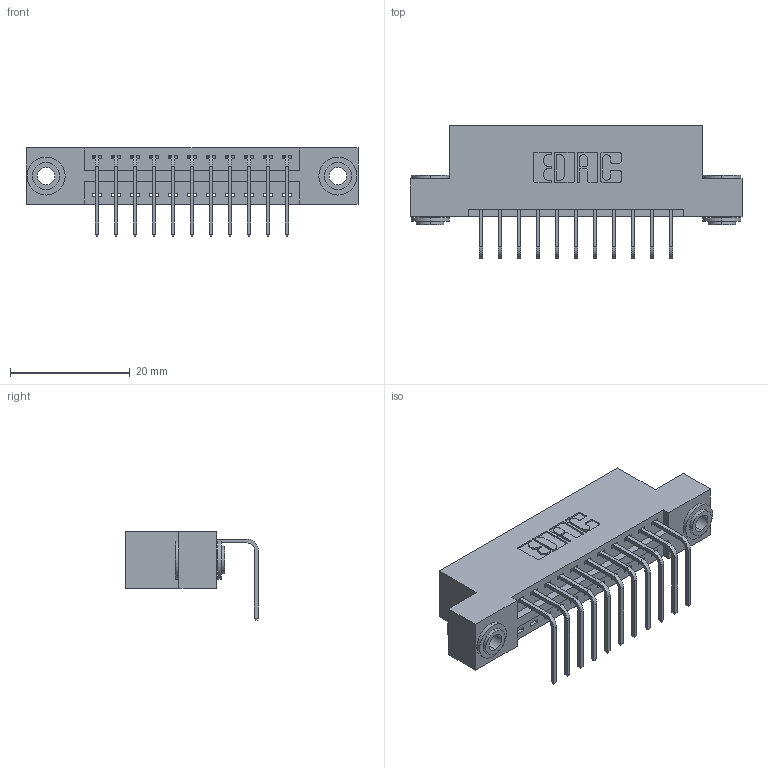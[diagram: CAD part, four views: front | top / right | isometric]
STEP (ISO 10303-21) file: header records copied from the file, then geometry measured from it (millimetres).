
FILE_DESCRIPTION (( 'STEP AP203' ), '1' );
FILE_NAME ('346-011-558-103.STEP', '2022-05-05T01:45:12', ( '' ), ( '' ), 'SwSTEP 2.0', 'SolidWorks 2020', '' );
FILE_SCHEMA (( 'CONFIG_CONTROL_DESIGN' ));
Length unit declared in the file: inch
Products named in the file (4): 345-250-002_345-250-002-102; 346 Part_Flush Mounting Lugs - 0.156 Dia-TH; 346-011-558-103; 345-292-001_558 Tail - 2
Assembly tree (14 placements, depth 2):
  346-011-558-103
    346 Part_Flush Mounting Lugs - 0.156 Dia-TH
    345-292-001_558 Tail - 2  x11
    345-250-002_345-250-002-102  x2
Bounding box: 55.5 x 22.16 x 14.73 mm (x, y, z)
Volume: 5136.8 mm3; surface area: 6556 mm2
Topology: 14 solids, 14 shells, 834 faces, 2443 edges, 1610 vertices
Faces by surface type: plane 562, cylinder 264, cone 8
Entity records: 12150 total; most frequent: CARTESIAN_POINT 2074, ORIENTED_EDGE 2010, DIRECTION 1897, EDGE_CURVE 1005, VECTOR 805, LINE 805, VERTEX_POINT 666, AXIS2_PLACEMENT_3D 546
